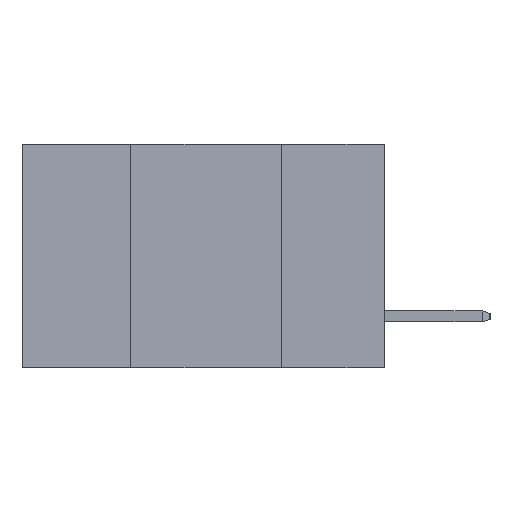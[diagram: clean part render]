
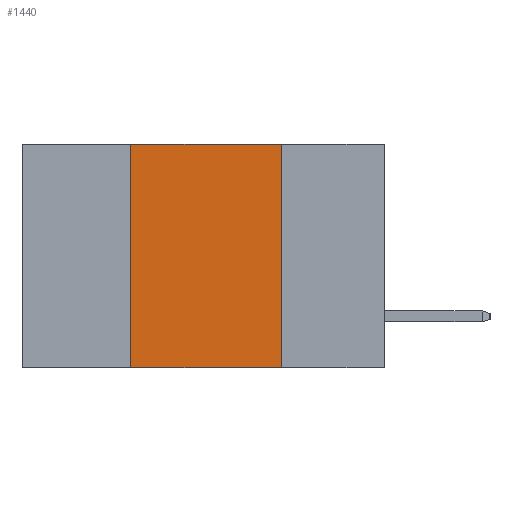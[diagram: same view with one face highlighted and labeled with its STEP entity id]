
A CAD part, left-side view. The second image highlights one B-rep face of the part: STEP entity #1440.
In plain terms, the highlighted planar face has unit normal (-1, 0, 0).
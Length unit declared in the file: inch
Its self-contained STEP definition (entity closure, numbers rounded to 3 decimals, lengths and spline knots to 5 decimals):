
#36 = LINE ( 'NONE', #5610, #10536 ) ;
#67 = ORIENTED_EDGE ( 'NONE', *, *, #4057, .F. ) ;
#278 = DIRECTION ( 'NONE',  ( 1., 0., 0. ) ) ;
#402 = AXIS2_PLACEMENT_3D ( 'NONE', #14859, #278, #12010 ) ;
#851 = VECTOR ( 'NONE', #3577, 39.37008 ) ;
#1067 = EDGE_CURVE ( 'NONE', #11907, #13929, #1298, .T. ) ;
#1298 = LINE ( 'NONE', #10213, #851 ) ;
#1440 = ADVANCED_FACE ( 'NONE', ( #15533 ), #9764, .F. ) ;
#1912 = VERTEX_POINT ( 'NONE', #16217 ) ;
#3320 = EDGE_CURVE ( 'NONE', #14602, #13929, #5633, .T. ) ;
#3373 = CARTESIAN_POINT ( 'NONE',  ( 0., 0.17, -0.37 ) ) ;
#3375 = EDGE_CURVE ( 'NONE', #1912, #14602, #36, .T. ) ;
#3577 = DIRECTION ( 'NONE',  ( 0., -1., 0. ) ) ;
#4057 = EDGE_CURVE ( 'NONE', #11907, #1912, #7857, .T. ) ;
#5610 = CARTESIAN_POINT ( 'NONE',  ( 0., 0.6, 0. ) ) ;
#5633 = LINE ( 'NONE', #6826, #8840 ) ;
#5782 = DIRECTION ( 'NONE',  ( 0., -1., 0. ) ) ;
#6637 = DIRECTION ( 'NONE',  ( 0., 0., -1. ) ) ;
#6739 = ORIENTED_EDGE ( 'NONE', *, *, #3320, .F. ) ;
#6826 = CARTESIAN_POINT ( 'NONE',  ( 0., 0.17, -0.37 ) ) ;
#7455 = VECTOR ( 'NONE', #14446, 39.37008 ) ;
#7496 = CARTESIAN_POINT ( 'NONE',  ( 0., 0.17, 0. ) ) ;
#7857 = LINE ( 'NONE', #13996, #7455 ) ;
#8669 = CARTESIAN_POINT ( 'NONE',  ( 0., 0.42, -0.37 ) ) ;
#8840 = VECTOR ( 'NONE', #6637, 39.37008 ) ;
#9576 = ORIENTED_EDGE ( 'NONE', *, *, #1067, .T. ) ;
#9764 = PLANE ( 'NONE',  #402 ) ;
#10213 = CARTESIAN_POINT ( 'NONE',  ( 0., 0.6, -0.37 ) ) ;
#10536 = VECTOR ( 'NONE', #5782, 39.37008 ) ;
#11385 = EDGE_LOOP ( 'NONE', ( #6739, #15091, #67, #9576 ) ) ;
#11907 = VERTEX_POINT ( 'NONE', #8669 ) ;
#12010 = DIRECTION ( 'NONE',  ( 0., 0., -1. ) ) ;
#13929 = VERTEX_POINT ( 'NONE', #3373 ) ;
#13996 = CARTESIAN_POINT ( 'NONE',  ( 0., 0.42, -0.37 ) ) ;
#14446 = DIRECTION ( 'NONE',  ( 0., 0., 1. ) ) ;
#14602 = VERTEX_POINT ( 'NONE', #7496 ) ;
#14859 = CARTESIAN_POINT ( 'NONE',  ( 0., 0.6, 0. ) ) ;
#15091 = ORIENTED_EDGE ( 'NONE', *, *, #3375, .F. ) ;
#15533 = FACE_OUTER_BOUND ( 'NONE', #11385, .T. ) ;
#16217 = CARTESIAN_POINT ( 'NONE',  ( 0., 0.42, 0. ) ) ;
